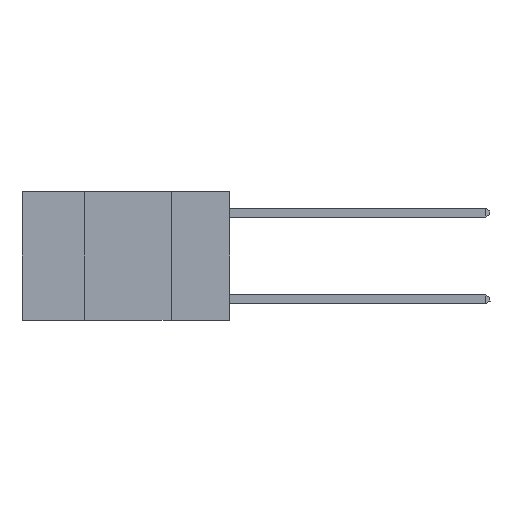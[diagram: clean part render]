
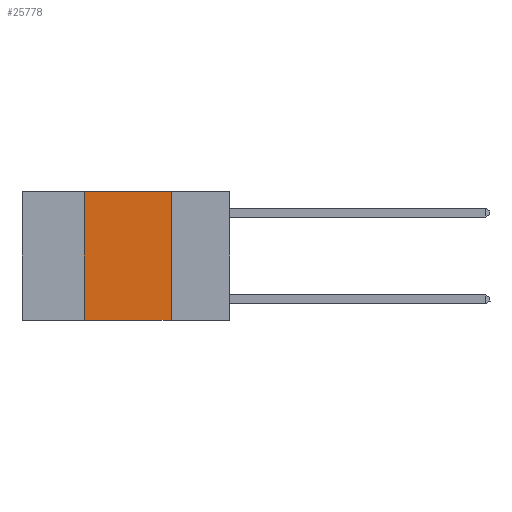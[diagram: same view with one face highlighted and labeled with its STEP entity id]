
A CAD part, left-side view. The second image highlights one B-rep face of the part: STEP entity #25778.
In plain terms, the highlighted planar face has unit normal (-1, 0, 0).
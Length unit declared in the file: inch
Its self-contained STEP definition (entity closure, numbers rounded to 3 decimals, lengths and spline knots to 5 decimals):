
#2682 = ORIENTED_EDGE ( 'NONE', *, *, #28140, .F. ) ;
#4225 = VECTOR ( 'NONE', #19641, 39.37008 ) ;
#4522 = LINE ( 'NONE', #22011, #20607 ) ;
#5079 = VERTEX_POINT ( 'NONE', #25736 ) ;
#5334 = FACE_OUTER_BOUND ( 'NONE', #7247, .T. ) ;
#5349 = CARTESIAN_POINT ( 'NONE',  ( 0., 0.6, 0. ) ) ;
#7247 = EDGE_LOOP ( 'NONE', ( #23491, #2682, #26694, #25689 ) ) ;
#7602 = PLANE ( 'NONE',  #13062 ) ;
#7677 = VERTEX_POINT ( 'NONE', #15575 ) ;
#8451 = VECTOR ( 'NONE', #18825, 39.37008 ) ;
#8970 = LINE ( 'NONE', #24136, #19837 ) ;
#9139 = LINE ( 'NONE', #12281, #8451 ) ;
#9813 = DIRECTION ( 'NONE',  ( 1., 0., 0. ) ) ;
#11128 = DIRECTION ( 'NONE',  ( 0., -1., 0. ) ) ;
#11351 = EDGE_CURVE ( 'NONE', #5079, #23879, #28083, .T. ) ;
#12281 = CARTESIAN_POINT ( 'NONE',  ( 0., 0.17, 0. ) ) ;
#13062 = AXIS2_PLACEMENT_3D ( 'NONE', #5349, #9813, #24997 ) ;
#13476 = VERTEX_POINT ( 'NONE', #22432 ) ;
#15575 = CARTESIAN_POINT ( 'NONE',  ( 0., 0.17, 0. ) ) ;
#16174 = CARTESIAN_POINT ( 'NONE',  ( 0., 0.42, 0. ) ) ;
#17427 = EDGE_CURVE ( 'NONE', #5079, #13476, #8970, .T. ) ;
#17467 = CARTESIAN_POINT ( 'NONE',  ( 0., 0.42, 0. ) ) ;
#18825 = DIRECTION ( 'NONE',  ( 0., 0., -1. ) ) ;
#19641 = DIRECTION ( 'NONE',  ( 0., 0., 1. ) ) ;
#19837 = VECTOR ( 'NONE', #11128, 39.37008 ) ;
#20607 = VECTOR ( 'NONE', #24197, 39.37008 ) ;
#22011 = CARTESIAN_POINT ( 'NONE',  ( 0., 0.6, 0. ) ) ;
#22432 = CARTESIAN_POINT ( 'NONE',  ( 0., 0.17, -0.37 ) ) ;
#23491 = ORIENTED_EDGE ( 'NONE', *, *, #25892, .F. ) ;
#23879 = VERTEX_POINT ( 'NONE', #16174 ) ;
#24136 = CARTESIAN_POINT ( 'NONE',  ( 0., 0.6, -0.37 ) ) ;
#24197 = DIRECTION ( 'NONE',  ( 0., -1., 0. ) ) ;
#24997 = DIRECTION ( 'NONE',  ( 0., 0., -1. ) ) ;
#25689 = ORIENTED_EDGE ( 'NONE', *, *, #17427, .T. ) ;
#25736 = CARTESIAN_POINT ( 'NONE',  ( 0., 0.42, -0.37 ) ) ;
#25778 = ADVANCED_FACE ( 'NONE', ( #5334 ), #7602, .F. ) ;
#25892 = EDGE_CURVE ( 'NONE', #7677, #13476, #9139, .T. ) ;
#26694 = ORIENTED_EDGE ( 'NONE', *, *, #11351, .F. ) ;
#28083 = LINE ( 'NONE', #17467, #4225 ) ;
#28140 = EDGE_CURVE ( 'NONE', #23879, #7677, #4522, .T. ) ;
